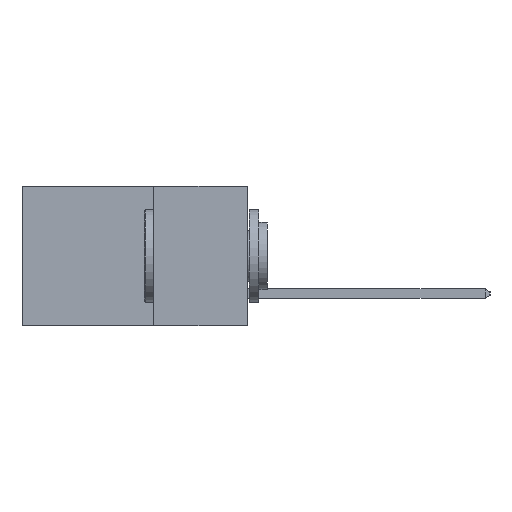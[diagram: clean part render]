
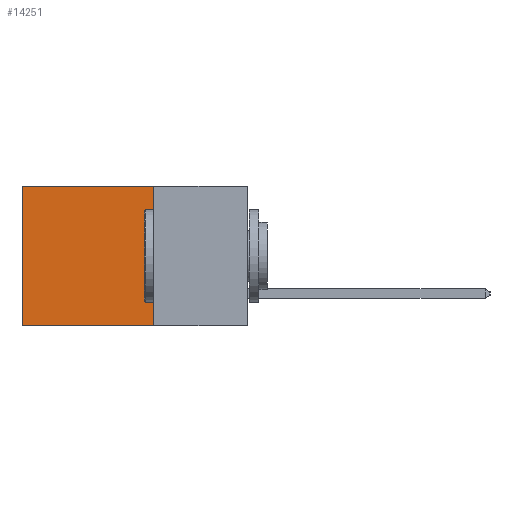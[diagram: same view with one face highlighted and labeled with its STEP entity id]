
A CAD part, left-side view. The second image highlights one B-rep face of the part: STEP entity #14251.
In plain terms, the highlighted planar face has unit normal (-1, 0, 0).
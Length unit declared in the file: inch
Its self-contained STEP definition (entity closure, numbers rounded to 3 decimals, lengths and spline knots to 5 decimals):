
#997 = VECTOR ( 'NONE', #3093, 39.37008 ) ;
#2632 = VERTEX_POINT ( 'NONE', #17441 ) ;
#3022 = ORIENTED_EDGE ( 'NONE', *, *, #16106, .F. ) ;
#3093 = DIRECTION ( 'NONE',  ( 0., 0., -1. ) ) ;
#3312 = CARTESIAN_POINT ( 'NONE',  ( 0.2615, 0.6, -0.37 ) ) ;
#5888 = LINE ( 'NONE', #3312, #997 ) ;
#5924 = CARTESIAN_POINT ( 'NONE',  ( 0.2615, 0.6, -0.37 ) ) ;
#6043 = CARTESIAN_POINT ( 'NONE',  ( 0.2615, 0.25, 0. ) ) ;
#6617 = CARTESIAN_POINT ( 'NONE',  ( 0.2615, 0.25, -0.37 ) ) ;
#7264 = LINE ( 'NONE', #15023, #21245 ) ;
#7339 = CARTESIAN_POINT ( 'NONE',  ( 0.2615, 0.6, 0. ) ) ;
#7446 = VERTEX_POINT ( 'NONE', #7339 ) ;
#8311 = DIRECTION ( 'NONE',  ( 0., 1., 0. ) ) ;
#9004 = EDGE_CURVE ( 'NONE', #21854, #2632, #7264, .T. ) ;
#10405 = VERTEX_POINT ( 'NONE', #5924 ) ;
#10588 = EDGE_CURVE ( 'NONE', #7446, #10405, #5888, .T. ) ;
#13065 = DIRECTION ( 'NONE',  ( 0., 0., -1. ) ) ;
#13106 = DIRECTION ( 'NONE',  ( 1., 0., 0. ) ) ;
#13236 = AXIS2_PLACEMENT_3D ( 'NONE', #13815, #13106, #13065 ) ;
#13679 = VECTOR ( 'NONE', #8311, 39.37008 ) ;
#13815 = CARTESIAN_POINT ( 'NONE',  ( 0.2615, 0.25, -0.37 ) ) ;
#13875 = PLANE ( 'NONE',  #13236 ) ;
#14251 = ADVANCED_FACE ( 'NONE', ( #16631 ), #13875, .F. ) ;
#14867 = ORIENTED_EDGE ( 'NONE', *, *, #10588, .T. ) ;
#15023 = CARTESIAN_POINT ( 'NONE',  ( 0.2615, 0.25, -0.37 ) ) ;
#15202 = DIRECTION ( 'NONE',  ( 0., 0., -1. ) ) ;
#15445 = ORIENTED_EDGE ( 'NONE', *, *, #20239, .T. ) ;
#15966 = VECTOR ( 'NONE', #21211, 39.37008 ) ;
#16106 = EDGE_CURVE ( 'NONE', #2632, #10405, #16548, .T. ) ;
#16482 = EDGE_LOOP ( 'NONE', ( #14867, #3022, #21307, #15445 ) ) ;
#16548 = LINE ( 'NONE', #6617, #15966 ) ;
#16631 = FACE_OUTER_BOUND ( 'NONE', #16482, .T. ) ;
#17441 = CARTESIAN_POINT ( 'NONE',  ( 0.2615, 0.25, -0.37 ) ) ;
#20239 = EDGE_CURVE ( 'NONE', #21854, #7446, #22702, .T. ) ;
#21211 = DIRECTION ( 'NONE',  ( 0., 1., 0. ) ) ;
#21245 = VECTOR ( 'NONE', #15202, 39.37008 ) ;
#21307 = ORIENTED_EDGE ( 'NONE', *, *, #9004, .F. ) ;
#21854 = VERTEX_POINT ( 'NONE', #6043 ) ;
#22702 = LINE ( 'NONE', #22835, #13679 ) ;
#22835 = CARTESIAN_POINT ( 'NONE',  ( 0.2615, 0.25, 0. ) ) ;
